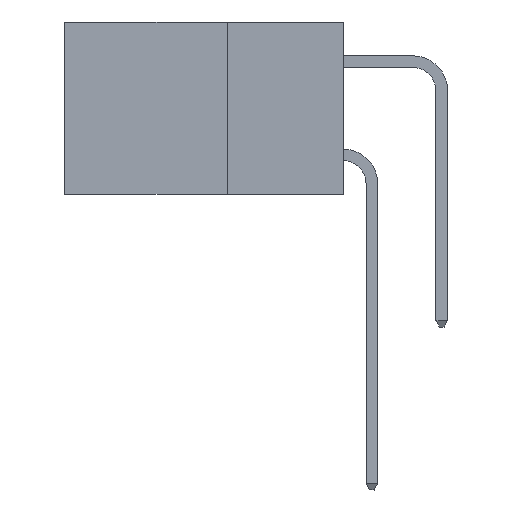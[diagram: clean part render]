
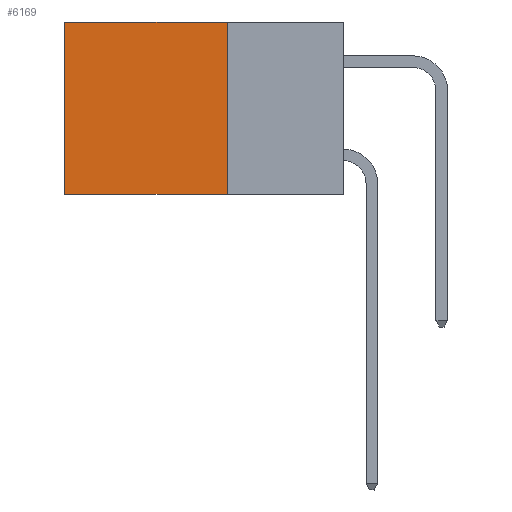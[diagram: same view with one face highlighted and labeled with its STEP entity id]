
A CAD part, left-side view. The second image highlights one B-rep face of the part: STEP entity #6169.
In plain terms, the highlighted planar face has unit normal (-1, 0, 0).
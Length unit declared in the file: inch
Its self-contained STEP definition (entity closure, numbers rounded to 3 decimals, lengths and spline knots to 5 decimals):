
#37 = CARTESIAN_POINT ( 'NONE',  ( 0.2615, 0.25, -0.37 ) ) ;
#122 = LINE ( 'NONE', #37, #7573 ) ;
#452 = EDGE_CURVE ( 'NONE', #8636, #5868, #6158, .T. ) ;
#972 = CARTESIAN_POINT ( 'NONE',  ( 0.2615, 0.25, -0.37 ) ) ;
#1240 = ORIENTED_EDGE ( 'NONE', *, *, #8526, .F. ) ;
#2708 = EDGE_LOOP ( 'NONE', ( #12500, #3373, #1240, #13427 ) ) ;
#3107 = VERTEX_POINT ( 'NONE', #11740 ) ;
#3301 = EDGE_CURVE ( 'NONE', #5868, #7476, #7512, .T. ) ;
#3373 = ORIENTED_EDGE ( 'NONE', *, *, #13586, .F. ) ;
#3939 = DIRECTION ( 'NONE',  ( 0., 0., -1. ) ) ;
#4146 = DIRECTION ( 'NONE',  ( 0., 1., 0. ) ) ;
#4173 = VECTOR ( 'NONE', #4146, 39.37008 ) ;
#4764 = AXIS2_PLACEMENT_3D ( 'NONE', #972, #10526, #5739 ) ;
#5462 = VECTOR ( 'NONE', #3939, 39.37008 ) ;
#5608 = CARTESIAN_POINT ( 'NONE',  ( 0.2615, 0.6, -0.37 ) ) ;
#5739 = DIRECTION ( 'NONE',  ( 0., 0., -1. ) ) ;
#5868 = VERTEX_POINT ( 'NONE', #11000 ) ;
#6158 = LINE ( 'NONE', #13360, #4173 ) ;
#6169 = ADVANCED_FACE ( 'NONE', ( #15078 ), #11677, .F. ) ;
#6964 = LINE ( 'NONE', #12837, #9791 ) ;
#7476 = VERTEX_POINT ( 'NONE', #12510 ) ;
#7512 = LINE ( 'NONE', #5608, #5462 ) ;
#7573 = VECTOR ( 'NONE', #11439, 39.37008 ) ;
#8526 = EDGE_CURVE ( 'NONE', #8636, #3107, #122, .T. ) ;
#8636 = VERTEX_POINT ( 'NONE', #9307 ) ;
#9161 = DIRECTION ( 'NONE',  ( 0., 1., 0. ) ) ;
#9307 = CARTESIAN_POINT ( 'NONE',  ( 0.2615, 0.25, 0. ) ) ;
#9791 = VECTOR ( 'NONE', #9161, 39.37008 ) ;
#10526 = DIRECTION ( 'NONE',  ( 1., 0., 0. ) ) ;
#11000 = CARTESIAN_POINT ( 'NONE',  ( 0.2615, 0.6, 0. ) ) ;
#11439 = DIRECTION ( 'NONE',  ( 0., 0., -1. ) ) ;
#11677 = PLANE ( 'NONE',  #4764 ) ;
#11740 = CARTESIAN_POINT ( 'NONE',  ( 0.2615, 0.25, -0.37 ) ) ;
#12500 = ORIENTED_EDGE ( 'NONE', *, *, #3301, .T. ) ;
#12510 = CARTESIAN_POINT ( 'NONE',  ( 0.2615, 0.6, -0.37 ) ) ;
#12837 = CARTESIAN_POINT ( 'NONE',  ( 0.2615, 0.25, -0.37 ) ) ;
#13360 = CARTESIAN_POINT ( 'NONE',  ( 0.2615, 0.25, 0. ) ) ;
#13427 = ORIENTED_EDGE ( 'NONE', *, *, #452, .T. ) ;
#13586 = EDGE_CURVE ( 'NONE', #3107, #7476, #6964, .T. ) ;
#15078 = FACE_OUTER_BOUND ( 'NONE', #2708, .T. ) ;
